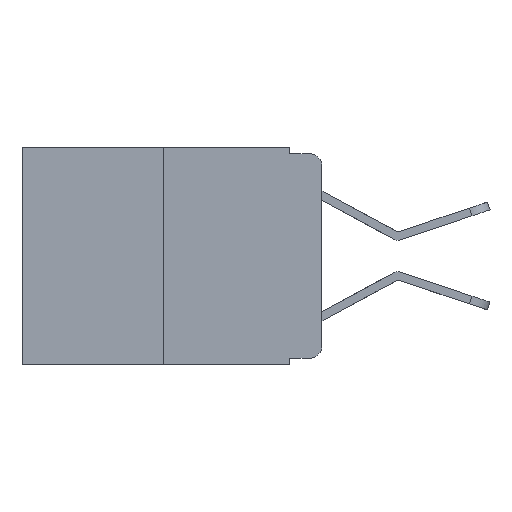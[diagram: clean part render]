
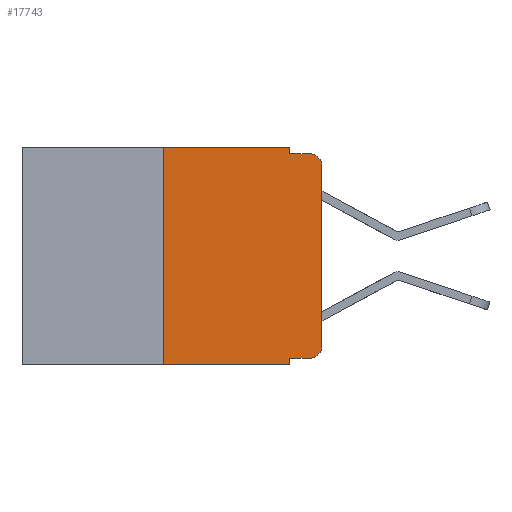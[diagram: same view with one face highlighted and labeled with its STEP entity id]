
A CAD part, left-side view. The second image highlights one B-rep face of the part: STEP entity #17743.
In plain terms, the highlighted planar face has unit normal (-1, 0, 0).
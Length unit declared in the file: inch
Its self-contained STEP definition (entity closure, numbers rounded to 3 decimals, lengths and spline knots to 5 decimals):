
#263 = AXIS2_PLACEMENT_3D ( 'NONE', #7575, #16093, #16387 ) ;
#408 = PLANE ( 'NONE',  #6853 ) ;
#578 = CARTESIAN_POINT ( 'NONE',  ( 0., 0.02, -0.333 ) ) ;
#624 = LINE ( 'NONE', #20715, #17004 ) ;
#679 = DIRECTION ( 'NONE',  ( 0., 0., 1. ) ) ;
#752 = ORIENTED_EDGE ( 'NONE', *, *, #11305, .F. ) ;
#825 = CARTESIAN_POINT ( 'NONE',  ( 0., 0.02, -0.01 ) ) ;
#939 = DIRECTION ( 'NONE',  ( -1., 0., 0. ) ) ;
#1476 = LINE ( 'NONE', #9956, #19465 ) ;
#2329 = FACE_OUTER_BOUND ( 'NONE', #8596, .T. ) ;
#3035 = EDGE_CURVE ( 'NONE', #20730, #8866, #12582, .T. ) ;
#3384 = CARTESIAN_POINT ( 'NONE',  ( 0., 0.473, -0.343 ) ) ;
#3423 = CARTESIAN_POINT ( 'NONE',  ( 0., 0.051, -0.343 ) ) ;
#3481 = EDGE_CURVE ( 'NONE', #8866, #4277, #6244, .T. ) ;
#3501 = VECTOR ( 'NONE', #10603, 39.37008 ) ;
#3518 = CARTESIAN_POINT ( 'NONE',  ( 0., 0.051, -0.01 ) ) ;
#3707 = ORIENTED_EDGE ( 'NONE', *, *, #6424, .F. ) ;
#3835 = LINE ( 'NONE', #9027, #4384 ) ;
#3880 = CARTESIAN_POINT ( 'NONE',  ( 0., 0.051, 0. ) ) ;
#4277 = VERTEX_POINT ( 'NONE', #825 ) ;
#4384 = VECTOR ( 'NONE', #10575, 39.37008 ) ;
#5320 = DIRECTION ( 'NONE',  ( 0., 0., -1. ) ) ;
#5554 = CARTESIAN_POINT ( 'NONE',  ( 0., 0.473, 0. ) ) ;
#6244 = LINE ( 'NONE', #3518, #3501 ) ;
#6312 = ORIENTED_EDGE ( 'NONE', *, *, #17369, .T. ) ;
#6424 = EDGE_CURVE ( 'NONE', #19310, #9986, #624, .T. ) ;
#6471 = ORIENTED_EDGE ( 'NONE', *, *, #3481, .F. ) ;
#6853 = AXIS2_PLACEMENT_3D ( 'NONE', #5554, #19321, #5320 ) ;
#6862 = DIRECTION ( 'NONE',  ( 0., 0., -1. ) ) ;
#7278 = VERTEX_POINT ( 'NONE', #14932 ) ;
#7575 = CARTESIAN_POINT ( 'NONE',  ( 0., 0.02, -0.03 ) ) ;
#8235 = VERTEX_POINT ( 'NONE', #22482 ) ;
#8308 = EDGE_CURVE ( 'NONE', #8235, #11902, #13117, .T. ) ;
#8485 = VECTOR ( 'NONE', #679, 39.37008 ) ;
#8596 = EDGE_LOOP ( 'NONE', ( #14795, #6312, #6471, #16496, #752, #3707, #9460, #18793, #17901, #18673 ) ) ;
#8866 = VERTEX_POINT ( 'NONE', #16601 ) ;
#9023 = VECTOR ( 'NONE', #10322, 39.37008 ) ;
#9027 = CARTESIAN_POINT ( 'NONE',  ( 0., 0.051, -0.333 ) ) ;
#9076 = LINE ( 'NONE', #13840, #15104 ) ;
#9095 = VERTEX_POINT ( 'NONE', #578 ) ;
#9460 = ORIENTED_EDGE ( 'NONE', *, *, #19906, .T. ) ;
#9956 = CARTESIAN_POINT ( 'NONE',  ( 0., 0.051, 0. ) ) ;
#9986 = VERTEX_POINT ( 'NONE', #13059 ) ;
#10120 = EDGE_CURVE ( 'NONE', #7278, #12039, #1476, .T. ) ;
#10166 = CARTESIAN_POINT ( 'NONE',  ( 0., 0., 0. ) ) ;
#10322 = DIRECTION ( 'NONE',  ( 0., -1., 0. ) ) ;
#10575 = DIRECTION ( 'NONE',  ( 0., -1., 0. ) ) ;
#10603 = DIRECTION ( 'NONE',  ( 0., -1., 0. ) ) ;
#11105 = CIRCLE ( 'NONE', #263, 0.02 ) ;
#11305 = EDGE_CURVE ( 'NONE', #9986, #20730, #9076, .T. ) ;
#11430 = DIRECTION ( 'NONE',  ( 0., 0., -1. ) ) ;
#11724 = DIRECTION ( 'NONE',  ( 0., 0., -1. ) ) ;
#11790 = LINE ( 'NONE', #3384, #9023 ) ;
#11902 = VERTEX_POINT ( 'NONE', #14826 ) ;
#12039 = VERTEX_POINT ( 'NONE', #3423 ) ;
#12217 = EDGE_CURVE ( 'NONE', #9095, #8235, #19119, .T. ) ;
#12582 = LINE ( 'NONE', #17283, #13939 ) ;
#13059 = CARTESIAN_POINT ( 'NONE',  ( 0., 0.25, 0. ) ) ;
#13117 = LINE ( 'NONE', #10166, #8485 ) ;
#13840 = CARTESIAN_POINT ( 'NONE',  ( 0., 0.473, 0. ) ) ;
#13939 = VECTOR ( 'NONE', #6862, 39.37008 ) ;
#14795 = ORIENTED_EDGE ( 'NONE', *, *, #8308, .T. ) ;
#14819 = CARTESIAN_POINT ( 'NONE',  ( 0., 0.02, -0.313 ) ) ;
#14826 = CARTESIAN_POINT ( 'NONE',  ( 0., 0., -0.03 ) ) ;
#14932 = CARTESIAN_POINT ( 'NONE',  ( 0., 0.051, -0.333 ) ) ;
#15104 = VECTOR ( 'NONE', #20683, 39.37008 ) ;
#16093 = DIRECTION ( 'NONE',  ( -1., 0., 0. ) ) ;
#16387 = DIRECTION ( 'NONE',  ( 0., 0., -1. ) ) ;
#16496 = ORIENTED_EDGE ( 'NONE', *, *, #3035, .F. ) ;
#16601 = CARTESIAN_POINT ( 'NONE',  ( 0., 0.051, -0.01 ) ) ;
#17002 = AXIS2_PLACEMENT_3D ( 'NONE', #14819, #939, #11430 ) ;
#17004 = VECTOR ( 'NONE', #22535, 39.37008 ) ;
#17283 = CARTESIAN_POINT ( 'NONE',  ( 0., 0.051, 0. ) ) ;
#17369 = EDGE_CURVE ( 'NONE', #11902, #4277, #11105, .T. ) ;
#17743 = ADVANCED_FACE ( 'NONE', ( #2329 ), #408, .F. ) ;
#17901 = ORIENTED_EDGE ( 'NONE', *, *, #21274, .T. ) ;
#18673 = ORIENTED_EDGE ( 'NONE', *, *, #12217, .T. ) ;
#18793 = ORIENTED_EDGE ( 'NONE', *, *, #10120, .F. ) ;
#19119 = CIRCLE ( 'NONE', #17002, 0.02 ) ;
#19310 = VERTEX_POINT ( 'NONE', #20878 ) ;
#19321 = DIRECTION ( 'NONE',  ( 1., 0., 0. ) ) ;
#19465 = VECTOR ( 'NONE', #11724, 39.37008 ) ;
#19906 = EDGE_CURVE ( 'NONE', #19310, #12039, #11790, .T. ) ;
#20683 = DIRECTION ( 'NONE',  ( 0., -1., 0. ) ) ;
#20715 = CARTESIAN_POINT ( 'NONE',  ( 0., 0.25, 0. ) ) ;
#20730 = VERTEX_POINT ( 'NONE', #3880 ) ;
#20878 = CARTESIAN_POINT ( 'NONE',  ( 0., 0.25, -0.343 ) ) ;
#21274 = EDGE_CURVE ( 'NONE', #7278, #9095, #3835, .T. ) ;
#22482 = CARTESIAN_POINT ( 'NONE',  ( 0., 0., -0.313 ) ) ;
#22535 = DIRECTION ( 'NONE',  ( 0., 0., 1. ) ) ;
